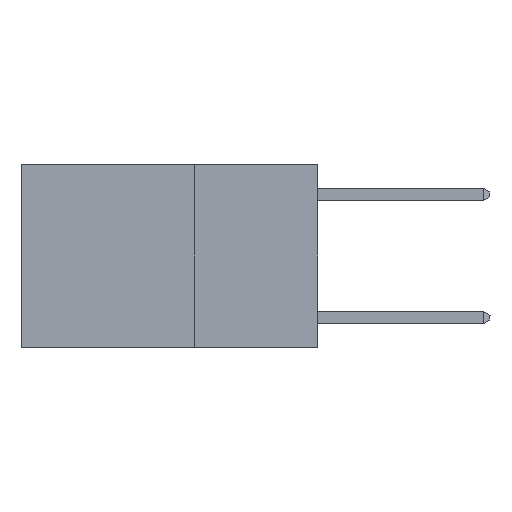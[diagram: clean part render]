
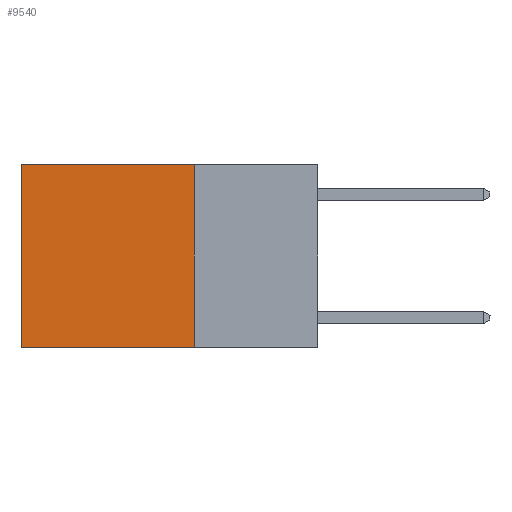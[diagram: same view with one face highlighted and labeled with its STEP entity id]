
A CAD part, left-side view. The second image highlights one B-rep face of the part: STEP entity #9540.
In plain terms, the highlighted planar face has unit normal (-1, 0, 0).
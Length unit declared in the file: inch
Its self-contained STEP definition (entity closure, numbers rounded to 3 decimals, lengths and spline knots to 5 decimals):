
#1 = VERTEX_POINT ( 'NONE', #18419 ) ;
#1320 = VECTOR ( 'NONE', #13729, 39.37008 ) ;
#1645 = EDGE_CURVE ( 'NONE', #1, #20078, #6762, .T. ) ;
#1690 = CARTESIAN_POINT ( 'NONE',  ( 0.2625, 0.25, 0. ) ) ;
#1837 = LINE ( 'NONE', #12166, #1320 ) ;
#1983 = EDGE_CURVE ( 'NONE', #1, #11469, #4982, .T. ) ;
#3228 = VERTEX_POINT ( 'NONE', #5527 ) ;
#4751 = CARTESIAN_POINT ( 'NONE',  ( 0.2625, 0.6, 0. ) ) ;
#4842 = CARTESIAN_POINT ( 'NONE',  ( 0.2625, 0.6, 0. ) ) ;
#4982 = LINE ( 'NONE', #16999, #16532 ) ;
#4998 = PLANE ( 'NONE',  #10912 ) ;
#5527 = CARTESIAN_POINT ( 'NONE',  ( 0.2625, 0.6, -0.37 ) ) ;
#6053 = DIRECTION ( 'NONE',  ( 0., 0., -1. ) ) ;
#6380 = DIRECTION ( 'NONE',  ( 0., 0., -1. ) ) ;
#6658 = FACE_OUTER_BOUND ( 'NONE', #10068, .T. ) ;
#6762 = LINE ( 'NONE', #6781, #7246 ) ;
#6781 = CARTESIAN_POINT ( 'NONE',  ( 0.2625, 0.25, 0. ) ) ;
#7246 = VECTOR ( 'NONE', #16171, 39.37008 ) ;
#7320 = LINE ( 'NONE', #4751, #19125 ) ;
#9216 = ORIENTED_EDGE ( 'NONE', *, *, #18608, .T. ) ;
#9456 = CARTESIAN_POINT ( 'NONE',  ( 0.2625, 0.25, -0.37 ) ) ;
#9540 = ADVANCED_FACE ( 'NONE', ( #6658 ), #4998, .F. ) ;
#9795 = DIRECTION ( 'NONE',  ( 0., 0., -1. ) ) ;
#10068 = EDGE_LOOP ( 'NONE', ( #9216, #13998, #10148, #16122 ) ) ;
#10148 = ORIENTED_EDGE ( 'NONE', *, *, #1983, .F. ) ;
#10912 = AXIS2_PLACEMENT_3D ( 'NONE', #1690, #18955, #9795 ) ;
#11469 = VERTEX_POINT ( 'NONE', #9456 ) ;
#12166 = CARTESIAN_POINT ( 'NONE',  ( 0.2625, 0.25, -0.37 ) ) ;
#13729 = DIRECTION ( 'NONE',  ( 0., 1., 0. ) ) ;
#13998 = ORIENTED_EDGE ( 'NONE', *, *, #16369, .F. ) ;
#16122 = ORIENTED_EDGE ( 'NONE', *, *, #1645, .T. ) ;
#16171 = DIRECTION ( 'NONE',  ( 0., 1., 0. ) ) ;
#16369 = EDGE_CURVE ( 'NONE', #11469, #3228, #1837, .T. ) ;
#16532 = VECTOR ( 'NONE', #6053, 39.37008 ) ;
#16999 = CARTESIAN_POINT ( 'NONE',  ( 0.2625, 0.25, 0. ) ) ;
#18419 = CARTESIAN_POINT ( 'NONE',  ( 0.2625, 0.25, 0. ) ) ;
#18608 = EDGE_CURVE ( 'NONE', #20078, #3228, #7320, .T. ) ;
#18955 = DIRECTION ( 'NONE',  ( 1., 0., 0. ) ) ;
#19125 = VECTOR ( 'NONE', #6380, 39.37008 ) ;
#20078 = VERTEX_POINT ( 'NONE', #4842 ) ;
